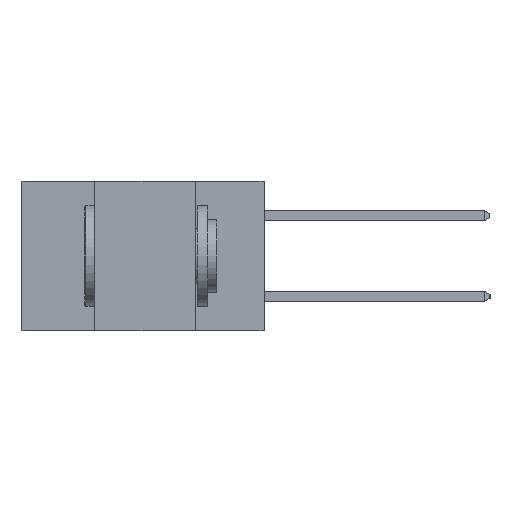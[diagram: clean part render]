
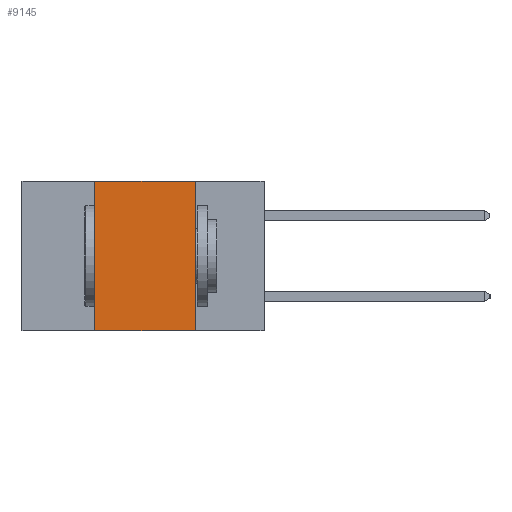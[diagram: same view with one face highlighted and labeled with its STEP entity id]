
A CAD part, left-side view. The second image highlights one B-rep face of the part: STEP entity #9145.
In plain terms, the highlighted planar face has unit normal (-1, 0, 0).
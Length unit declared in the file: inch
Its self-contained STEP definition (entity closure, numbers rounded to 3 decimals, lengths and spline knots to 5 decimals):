
#614 = EDGE_LOOP ( 'NONE', ( #7394, #2025, #15156, #10119 ) ) ;
#691 = DIRECTION ( 'NONE',  ( 0., 0., 1. ) ) ;
#962 = FACE_OUTER_BOUND ( 'NONE', #614, .T. ) ;
#1061 = EDGE_CURVE ( 'NONE', #12011, #10105, #14491, .T. ) ;
#1681 = EDGE_CURVE ( 'NONE', #8132, #10105, #5186, .T. ) ;
#1943 = VECTOR ( 'NONE', #14154, 39.37008 ) ;
#2025 = ORIENTED_EDGE ( 'NONE', *, *, #13578, .F. ) ;
#2514 = CARTESIAN_POINT ( 'NONE',  ( 0., 0.6, 0. ) ) ;
#3634 = AXIS2_PLACEMENT_3D ( 'NONE', #2514, #13628, #6203 ) ;
#5186 = LINE ( 'NONE', #10651, #1943 ) ;
#6203 = DIRECTION ( 'NONE',  ( 0., 0., -1. ) ) ;
#6910 = EDGE_CURVE ( 'NONE', #8132, #12605, #9020, .T. ) ;
#6917 = CARTESIAN_POINT ( 'NONE',  ( 0., 0.42, 0. ) ) ;
#7394 = ORIENTED_EDGE ( 'NONE', *, *, #1061, .F. ) ;
#7898 = VECTOR ( 'NONE', #11099, 39.37008 ) ;
#8132 = VERTEX_POINT ( 'NONE', #13574 ) ;
#8321 = VECTOR ( 'NONE', #15363, 39.37008 ) ;
#8710 = LINE ( 'NONE', #9199, #8321 ) ;
#9020 = LINE ( 'NONE', #12965, #11886 ) ;
#9145 = ADVANCED_FACE ( 'NONE', ( #962 ), #12375, .F. ) ;
#9199 = CARTESIAN_POINT ( 'NONE',  ( 0., 0.6, 0. ) ) ;
#9634 = CARTESIAN_POINT ( 'NONE',  ( 0., 0.17, -0.37 ) ) ;
#10105 = VERTEX_POINT ( 'NONE', #9634 ) ;
#10119 = ORIENTED_EDGE ( 'NONE', *, *, #1681, .T. ) ;
#10227 = CARTESIAN_POINT ( 'NONE',  ( 0., 0.17, -0.37 ) ) ;
#10651 = CARTESIAN_POINT ( 'NONE',  ( 0., 0.6, -0.37 ) ) ;
#11099 = DIRECTION ( 'NONE',  ( 0., 0., -1. ) ) ;
#11886 = VECTOR ( 'NONE', #691, 39.37008 ) ;
#12011 = VERTEX_POINT ( 'NONE', #15818 ) ;
#12375 = PLANE ( 'NONE',  #3634 ) ;
#12605 = VERTEX_POINT ( 'NONE', #6917 ) ;
#12965 = CARTESIAN_POINT ( 'NONE',  ( 0., 0.42, -0.37 ) ) ;
#13574 = CARTESIAN_POINT ( 'NONE',  ( 0., 0.42, -0.37 ) ) ;
#13578 = EDGE_CURVE ( 'NONE', #12605, #12011, #8710, .T. ) ;
#13628 = DIRECTION ( 'NONE',  ( 1., 0., 0. ) ) ;
#14154 = DIRECTION ( 'NONE',  ( 0., -1., 0. ) ) ;
#14491 = LINE ( 'NONE', #10227, #7898 ) ;
#15156 = ORIENTED_EDGE ( 'NONE', *, *, #6910, .F. ) ;
#15363 = DIRECTION ( 'NONE',  ( 0., -1., 0. ) ) ;
#15818 = CARTESIAN_POINT ( 'NONE',  ( 0., 0.17, 0. ) ) ;
